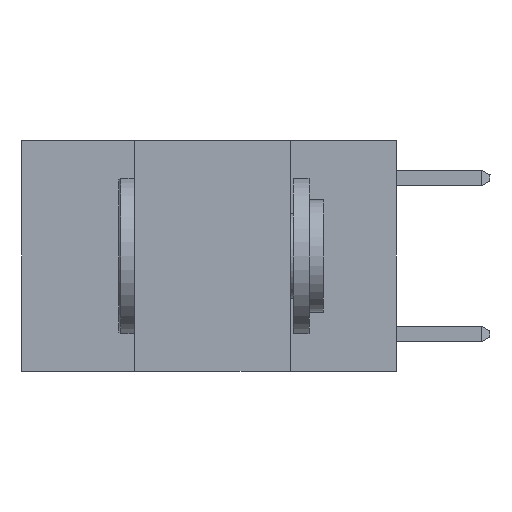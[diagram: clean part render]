
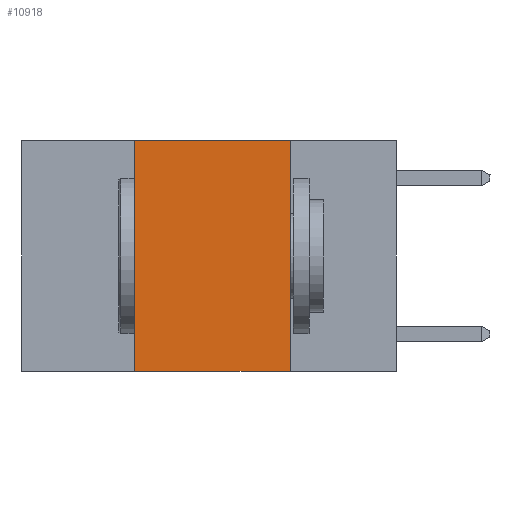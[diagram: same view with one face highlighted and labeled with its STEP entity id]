
A CAD part, left-side view. The second image highlights one B-rep face of the part: STEP entity #10918.
In plain terms, the highlighted planar face has unit normal (-1, 0, 0).
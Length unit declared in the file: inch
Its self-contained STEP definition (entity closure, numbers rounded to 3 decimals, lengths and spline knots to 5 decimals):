
#354 = VERTEX_POINT ( 'NONE', #2400 ) ;
#1231 = DIRECTION ( 'NONE',  ( 0., -1., 0. ) ) ;
#2105 = ORIENTED_EDGE ( 'NONE', *, *, #7932, .F. ) ;
#2115 = CARTESIAN_POINT ( 'NONE',  ( 0., 0.42, 0. ) ) ;
#2400 = CARTESIAN_POINT ( 'NONE',  ( 0., 0.17, -0.37 ) ) ;
#2883 = DIRECTION ( 'NONE',  ( 0., 0., -1. ) ) ;
#3792 = VERTEX_POINT ( 'NONE', #11698 ) ;
#4064 = VERTEX_POINT ( 'NONE', #7281 ) ;
#4105 = DIRECTION ( 'NONE',  ( 0., -1., 0. ) ) ;
#5823 = VECTOR ( 'NONE', #7693, 39.37008 ) ;
#6403 = CARTESIAN_POINT ( 'NONE',  ( 0., 0.17, 0. ) ) ;
#6933 = CARTESIAN_POINT ( 'NONE',  ( 0., 0.6, 0. ) ) ;
#7281 = CARTESIAN_POINT ( 'NONE',  ( 0., 0.42, -0.37 ) ) ;
#7348 = PLANE ( 'NONE',  #8956 ) ;
#7604 = VECTOR ( 'NONE', #2883, 39.37008 ) ;
#7693 = DIRECTION ( 'NONE',  ( 0., 0., 1. ) ) ;
#7932 = EDGE_CURVE ( 'NONE', #17204, #3792, #14978, .T. ) ;
#8673 = EDGE_LOOP ( 'NONE', ( #14351, #2105, #22049, #18537 ) ) ;
#8897 = CARTESIAN_POINT ( 'NONE',  ( 0., 0.6, -0.37 ) ) ;
#8956 = AXIS2_PLACEMENT_3D ( 'NONE', #6933, #15355, #20461 ) ;
#10918 = ADVANCED_FACE ( 'NONE', ( #11933 ), #7348, .F. ) ;
#11225 = CARTESIAN_POINT ( 'NONE',  ( 0., 0.6, 0. ) ) ;
#11639 = LINE ( 'NONE', #6403, #7604 ) ;
#11698 = CARTESIAN_POINT ( 'NONE',  ( 0., 0.17, 0. ) ) ;
#11933 = FACE_OUTER_BOUND ( 'NONE', #8673, .T. ) ;
#12346 = VECTOR ( 'NONE', #4105, 39.37008 ) ;
#14351 = ORIENTED_EDGE ( 'NONE', *, *, #19991, .F. ) ;
#14978 = LINE ( 'NONE', #11225, #18120 ) ;
#15355 = DIRECTION ( 'NONE',  ( 1., 0., 0. ) ) ;
#17204 = VERTEX_POINT ( 'NONE', #21234 ) ;
#17862 = LINE ( 'NONE', #8897, #12346 ) ;
#17929 = LINE ( 'NONE', #2115, #5823 ) ;
#18120 = VECTOR ( 'NONE', #1231, 39.37008 ) ;
#18537 = ORIENTED_EDGE ( 'NONE', *, *, #20287, .T. ) ;
#19991 = EDGE_CURVE ( 'NONE', #3792, #354, #11639, .T. ) ;
#20287 = EDGE_CURVE ( 'NONE', #4064, #354, #17862, .T. ) ;
#20461 = DIRECTION ( 'NONE',  ( 0., 0., -1. ) ) ;
#20752 = EDGE_CURVE ( 'NONE', #4064, #17204, #17929, .T. ) ;
#21234 = CARTESIAN_POINT ( 'NONE',  ( 0., 0.42, 0. ) ) ;
#22049 = ORIENTED_EDGE ( 'NONE', *, *, #20752, .F. ) ;
